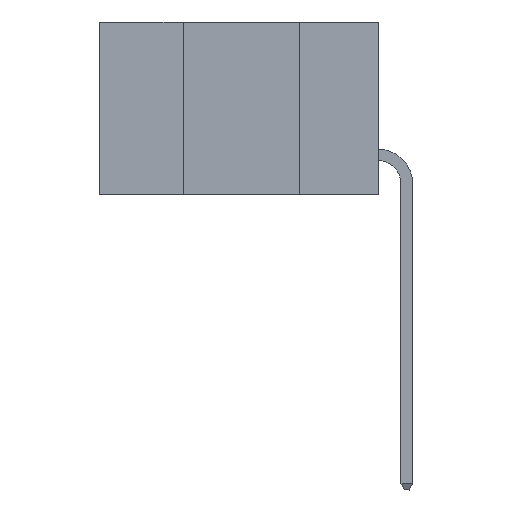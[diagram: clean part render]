
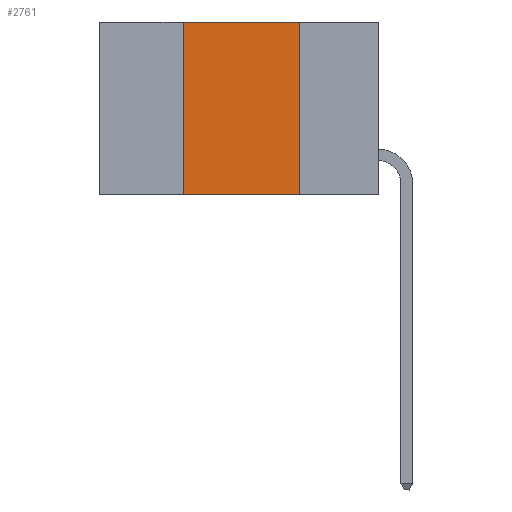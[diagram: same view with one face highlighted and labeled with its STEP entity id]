
A CAD part, left-side view. The second image highlights one B-rep face of the part: STEP entity #2761.
In plain terms, the highlighted planar face has unit normal (-1, 0, 0).
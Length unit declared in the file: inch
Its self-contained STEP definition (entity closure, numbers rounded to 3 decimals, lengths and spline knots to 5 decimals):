
#49 = CARTESIAN_POINT ( 'NONE',  ( 0., 0.42, -0.37 ) ) ;
#239 = CARTESIAN_POINT ( 'NONE',  ( 0., 0.42, -0.37 ) ) ;
#412 = ORIENTED_EDGE ( 'NONE', *, *, #2057, .T. ) ;
#415 = CARTESIAN_POINT ( 'NONE',  ( 0., 0.17, -0.37 ) ) ;
#942 = EDGE_CURVE ( 'NONE', #7968, #9053, #1317, .T. ) ;
#1317 = LINE ( 'NONE', #7269, #8770 ) ;
#1421 = CARTESIAN_POINT ( 'NONE',  ( 0., 0.6, 0. ) ) ;
#2057 = EDGE_CURVE ( 'NONE', #9287, #9053, #2485, .T. ) ;
#2485 = LINE ( 'NONE', #6850, #7709 ) ;
#2761 = ADVANCED_FACE ( 'NONE', ( #3398 ), #4978, .F. ) ;
#2936 = CARTESIAN_POINT ( 'NONE',  ( 0., 0.42, 0. ) ) ;
#2992 = ORIENTED_EDGE ( 'NONE', *, *, #3882, .F. ) ;
#3398 = FACE_OUTER_BOUND ( 'NONE', #7498, .T. ) ;
#3518 = DIRECTION ( 'NONE',  ( 0., 0., -1. ) ) ;
#3815 = DIRECTION ( 'NONE',  ( 0., -1., 0. ) ) ;
#3882 = EDGE_CURVE ( 'NONE', #5142, #7968, #9691, .T. ) ;
#4511 = LINE ( 'NONE', #49, #8281 ) ;
#4931 = CARTESIAN_POINT ( 'NONE',  ( 0., 0.6, 0. ) ) ;
#4978 = PLANE ( 'NONE',  #5310 ) ;
#5142 = VERTEX_POINT ( 'NONE', #2936 ) ;
#5310 = AXIS2_PLACEMENT_3D ( 'NONE', #4931, #6470, #8830 ) ;
#5392 = EDGE_CURVE ( 'NONE', #9287, #5142, #4511, .T. ) ;
#6410 = VECTOR ( 'NONE', #6678, 39.37008 ) ;
#6470 = DIRECTION ( 'NONE',  ( 1., 0., 0. ) ) ;
#6678 = DIRECTION ( 'NONE',  ( 0., -1., 0. ) ) ;
#6850 = CARTESIAN_POINT ( 'NONE',  ( 0., 0.6, -0.37 ) ) ;
#7269 = CARTESIAN_POINT ( 'NONE',  ( 0., 0.17, -0.37 ) ) ;
#7498 = EDGE_LOOP ( 'NONE', ( #8119, #2992, #9050, #412 ) ) ;
#7707 = CARTESIAN_POINT ( 'NONE',  ( 0., 0.17, 0. ) ) ;
#7709 = VECTOR ( 'NONE', #3815, 39.37008 ) ;
#7968 = VERTEX_POINT ( 'NONE', #7707 ) ;
#8119 = ORIENTED_EDGE ( 'NONE', *, *, #942, .F. ) ;
#8281 = VECTOR ( 'NONE', #9068, 39.37008 ) ;
#8770 = VECTOR ( 'NONE', #3518, 39.37008 ) ;
#8830 = DIRECTION ( 'NONE',  ( 0., 0., -1. ) ) ;
#9050 = ORIENTED_EDGE ( 'NONE', *, *, #5392, .F. ) ;
#9053 = VERTEX_POINT ( 'NONE', #415 ) ;
#9068 = DIRECTION ( 'NONE',  ( 0., 0., 1. ) ) ;
#9287 = VERTEX_POINT ( 'NONE', #239 ) ;
#9691 = LINE ( 'NONE', #1421, #6410 ) ;
